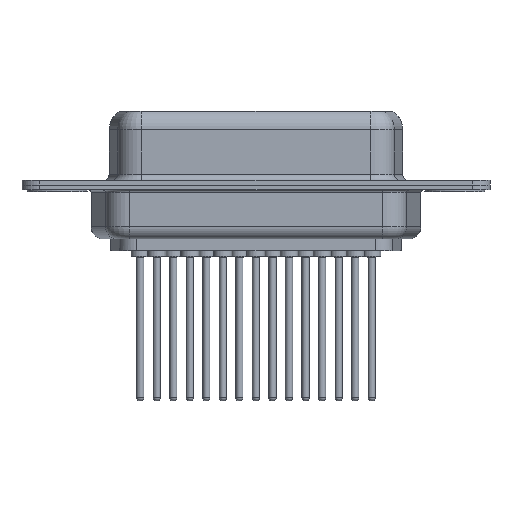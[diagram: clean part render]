
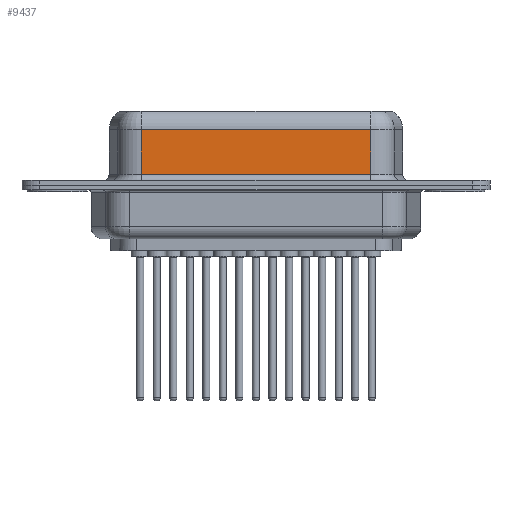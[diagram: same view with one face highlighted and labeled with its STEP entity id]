
A CAD part, front view. The second image highlights one B-rep face of the part: STEP entity #9437.
In plain terms, the highlighted planar face has unit normal (0, -1, 0).
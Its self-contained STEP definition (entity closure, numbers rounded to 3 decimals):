
#425 = VERTEX_POINT ( 'NONE', #9661 ) ;
#546 = CARTESIAN_POINT ( 'NONE',  ( 26.262, -3.95, 4.65 ) ) ;
#577 = CARTESIAN_POINT ( 'NONE',  ( 7.038, -3.95, 4.65 ) ) ;
#1121 = CARTESIAN_POINT ( 'NONE',  ( 26.262, -3.95, 6.4 ) ) ;
#1334 = PLANE ( 'NONE',  #14127 ) ;
#2301 = CARTESIAN_POINT ( 'NONE',  ( 26.262, -3.95, 4.65 ) ) ;
#3343 = VERTEX_POINT ( 'NONE', #13602 ) ;
#3486 = DIRECTION ( 'NONE',  ( 0., 0., -1. ) ) ;
#3564 = DIRECTION ( 'NONE',  ( 1., 0., 0. ) ) ;
#3618 = DIRECTION ( 'NONE',  ( -1., 0., 0. ) ) ;
#4437 = EDGE_CURVE ( 'NONE', #5322, #8397, #9739, .T. ) ;
#4908 = VECTOR ( 'NONE', #3486, 1000. ) ;
#5322 = VERTEX_POINT ( 'NONE', #546 ) ;
#5851 = DIRECTION ( 'NONE',  ( -1., 0., 0. ) ) ;
#5907 = EDGE_CURVE ( 'NONE', #3343, #425, #8629, .T. ) ;
#6386 = VECTOR ( 'NONE', #3564, 1000. ) ;
#7283 = LINE ( 'NONE', #1121, #12897 ) ;
#7480 = FACE_OUTER_BOUND ( 'NONE', #13492, .T. ) ;
#7587 = EDGE_CURVE ( 'NONE', #5322, #425, #7283, .T. ) ;
#7802 = EDGE_CURVE ( 'NONE', #8397, #3343, #8138, .T. ) ;
#8138 = LINE ( 'NONE', #14406, #4908 ) ;
#8397 = VERTEX_POINT ( 'NONE', #577 ) ;
#8629 = LINE ( 'NONE', #14646, #6386 ) ;
#9437 = ADVANCED_FACE ( 'NONE', ( #7480 ), #1334, .F. ) ;
#9661 = CARTESIAN_POINT ( 'NONE',  ( 26.262, -3.95, 0.9 ) ) ;
#9739 = LINE ( 'NONE', #2301, #9947 ) ;
#9807 = ORIENTED_EDGE ( 'NONE', *, *, #7802, .T. ) ;
#9947 = VECTOR ( 'NONE', #5851, 1000. ) ;
#11211 = CARTESIAN_POINT ( 'NONE',  ( 26.262, -3.95, 6.4 ) ) ;
#12650 = ORIENTED_EDGE ( 'NONE', *, *, #5907, .T. ) ;
#12793 = ORIENTED_EDGE ( 'NONE', *, *, #7587, .F. ) ;
#12897 = VECTOR ( 'NONE', #15935, 1000. ) ;
#13492 = EDGE_LOOP ( 'NONE', ( #12793, #14070, #9807, #12650 ) ) ;
#13602 = CARTESIAN_POINT ( 'NONE',  ( 7.038, -3.95, 0.9 ) ) ;
#13808 = DIRECTION ( 'NONE',  ( 0., 1., 0. ) ) ;
#14070 = ORIENTED_EDGE ( 'NONE', *, *, #4437, .T. ) ;
#14127 = AXIS2_PLACEMENT_3D ( 'NONE', #11211, #13808, #3618 ) ;
#14406 = CARTESIAN_POINT ( 'NONE',  ( 7.038, -3.95, 6.4 ) ) ;
#14646 = CARTESIAN_POINT ( 'NONE',  ( 26.262, -3.95, 0.9 ) ) ;
#15935 = DIRECTION ( 'NONE',  ( 0., 0., -1. ) ) ;
